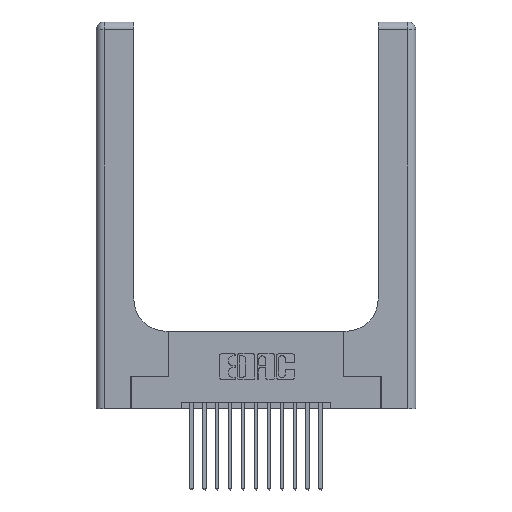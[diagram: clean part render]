
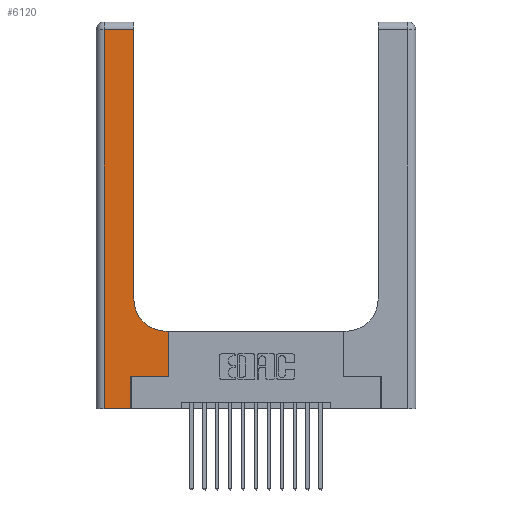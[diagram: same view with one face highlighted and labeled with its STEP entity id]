
A CAD part, top view. The second image highlights one B-rep face of the part: STEP entity #6120.
In plain terms, the highlighted planar face has unit normal (0, 0, 1).
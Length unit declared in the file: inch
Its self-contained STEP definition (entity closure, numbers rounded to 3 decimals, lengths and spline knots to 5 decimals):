
#691 = DIRECTION ( 'NONE',  ( -1., 0., 0. ) ) ;
#848 = EDGE_CURVE ( 'NONE', #15221, #10775, #6464, .T. ) ;
#928 = CARTESIAN_POINT ( 'NONE',  ( 0.2915, 2.94, 0.37 ) ) ;
#1224 = DIRECTION ( 'NONE',  ( 1., 0., 0. ) ) ;
#1626 = CARTESIAN_POINT ( 'NONE',  ( 0.5585, 0.6, 0.37 ) ) ;
#1683 = ORIENTED_EDGE ( 'NONE', *, *, #11446, .T. ) ;
#1730 = DIRECTION ( 'NONE',  ( 0., -1., 0. ) ) ;
#1877 = DIRECTION ( 'NONE',  ( -1., 0., 0. ) ) ;
#2250 = CIRCLE ( 'NONE', #7409, 0.25 ) ;
#2479 = VECTOR ( 'NONE', #5836, 39.37008 ) ;
#3103 = EDGE_LOOP ( 'NONE', ( #7829, #4779, #5491, #4378, #1683, #12751, #6017, #5024, #5542 ) ) ;
#3137 = CARTESIAN_POINT ( 'NONE',  ( 0.5415, 0.6, 0.37 ) ) ;
#3191 = CARTESIAN_POINT ( 'NONE',  ( 0.06, 3., 0.37 ) ) ;
#3253 = VECTOR ( 'NONE', #7052, 39.37008 ) ;
#3623 = CARTESIAN_POINT ( 'NONE',  ( 0., 2.94, 0.37 ) ) ;
#4041 = LINE ( 'NONE', #9307, #14291 ) ;
#4232 = CARTESIAN_POINT ( 'NONE',  ( 0.2915, 0.85, 0.37 ) ) ;
#4348 = DIRECTION ( 'NONE',  ( 1., 0., 0. ) ) ;
#4365 = CARTESIAN_POINT ( 'NONE',  ( 0.5585, 0.25, 0.37 ) ) ;
#4378 = ORIENTED_EDGE ( 'NONE', *, *, #6734, .T. ) ;
#4634 = EDGE_CURVE ( 'NONE', #12927, #4696, #2250, .T. ) ;
#4696 = VERTEX_POINT ( 'NONE', #4232 ) ;
#4779 = ORIENTED_EDGE ( 'NONE', *, *, #10586, .T. ) ;
#5024 = ORIENTED_EDGE ( 'NONE', *, *, #15710, .T. ) ;
#5060 = VERTEX_POINT ( 'NONE', #12260 ) ;
#5326 = EDGE_CURVE ( 'NONE', #5980, #5060, #13916, .T. ) ;
#5491 = ORIENTED_EDGE ( 'NONE', *, *, #848, .T. ) ;
#5542 = ORIENTED_EDGE ( 'NONE', *, *, #4634, .T. ) ;
#5788 = CARTESIAN_POINT ( 'NONE',  ( 0., 3., 0.37 ) ) ;
#5836 = DIRECTION ( 'NONE',  ( 0., 1., 0. ) ) ;
#5980 = VERTEX_POINT ( 'NONE', #16629 ) ;
#6017 = ORIENTED_EDGE ( 'NONE', *, *, #16628, .T. ) ;
#6120 = ADVANCED_FACE ( 'NONE', ( #12407 ), #14480, .F. ) ;
#6195 = LINE ( 'NONE', #3623, #16313 ) ;
#6464 = LINE ( 'NONE', #3191, #12597 ) ;
#6734 = EDGE_CURVE ( 'NONE', #10775, #13007, #4041, .T. ) ;
#6956 = CARTESIAN_POINT ( 'NONE',  ( 0.06, 0., 0.37 ) ) ;
#7042 = LINE ( 'NONE', #15326, #3253 ) ;
#7052 = DIRECTION ( 'NONE',  ( 0., 1., 0. ) ) ;
#7171 = CARTESIAN_POINT ( 'NONE',  ( 0.269, 0.25, 0.37 ) ) ;
#7409 = AXIS2_PLACEMENT_3D ( 'NONE', #17878, #9742, #1224 ) ;
#7829 = ORIENTED_EDGE ( 'NONE', *, *, #17960, .T. ) ;
#7991 = VECTOR ( 'NONE', #12187, 39.37008 ) ;
#8034 = CARTESIAN_POINT ( 'NONE',  ( 0.06, 2.94, 0.37 ) ) ;
#9150 = DIRECTION ( 'NONE',  ( -1., 0., 0. ) ) ;
#9307 = CARTESIAN_POINT ( 'NONE',  ( 0., 0., 0.37 ) ) ;
#9742 = DIRECTION ( 'NONE',  ( 0., 0., -1. ) ) ;
#9999 = LINE ( 'NONE', #4365, #2479 ) ;
#10367 = DIRECTION ( 'NONE',  ( 0., 0., -1. ) ) ;
#10384 = LINE ( 'NONE', #10767, #7991 ) ;
#10586 = EDGE_CURVE ( 'NONE', #13848, #15221, #6195, .T. ) ;
#10717 = DIRECTION ( 'NONE',  ( 1., 0., 0. ) ) ;
#10767 = CARTESIAN_POINT ( 'NONE',  ( 0.2915, 3., 0.37 ) ) ;
#10775 = VERTEX_POINT ( 'NONE', #6956 ) ;
#10956 = VERTEX_POINT ( 'NONE', #1626 ) ;
#11446 = EDGE_CURVE ( 'NONE', #13007, #5980, #7042, .T. ) ;
#12187 = DIRECTION ( 'NONE',  ( 0., 1., 0. ) ) ;
#12260 = CARTESIAN_POINT ( 'NONE',  ( 0.5585, 0.25, 0.37 ) ) ;
#12407 = FACE_OUTER_BOUND ( 'NONE', #3103, .T. ) ;
#12597 = VECTOR ( 'NONE', #1730, 39.37008 ) ;
#12751 = ORIENTED_EDGE ( 'NONE', *, *, #5326, .T. ) ;
#12927 = VERTEX_POINT ( 'NONE', #3137 ) ;
#13007 = VERTEX_POINT ( 'NONE', #13157 ) ;
#13157 = CARTESIAN_POINT ( 'NONE',  ( 0.269, 0., 0.37 ) ) ;
#13848 = VERTEX_POINT ( 'NONE', #928 ) ;
#13916 = LINE ( 'NONE', #7171, #14340 ) ;
#14283 = VECTOR ( 'NONE', #9150, 39.37008 ) ;
#14291 = VECTOR ( 'NONE', #10717, 39.37008 ) ;
#14340 = VECTOR ( 'NONE', #4348, 39.37008 ) ;
#14393 = AXIS2_PLACEMENT_3D ( 'NONE', #5788, #10367, #1877 ) ;
#14480 = PLANE ( 'NONE',  #14393 ) ;
#15221 = VERTEX_POINT ( 'NONE', #8034 ) ;
#15326 = CARTESIAN_POINT ( 'NONE',  ( 0.269, 0., 0.37 ) ) ;
#15710 = EDGE_CURVE ( 'NONE', #10956, #12927, #17373, .T. ) ;
#16313 = VECTOR ( 'NONE', #691, 39.37008 ) ;
#16628 = EDGE_CURVE ( 'NONE', #5060, #10956, #9999, .T. ) ;
#16629 = CARTESIAN_POINT ( 'NONE',  ( 0.269, 0.25, 0.37 ) ) ;
#17313 = CARTESIAN_POINT ( 'NONE',  ( 0.2915, 0.6, 0.37 ) ) ;
#17373 = LINE ( 'NONE', #17313, #14283 ) ;
#17878 = CARTESIAN_POINT ( 'NONE',  ( 0.5415, 0.85, 0.37 ) ) ;
#17960 = EDGE_CURVE ( 'NONE', #4696, #13848, #10384, .T. ) ;
